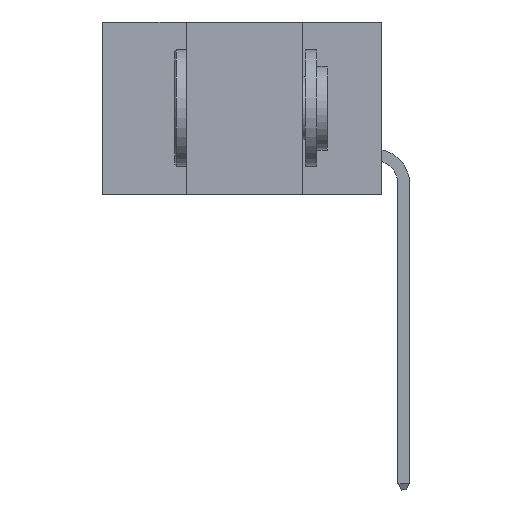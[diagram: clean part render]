
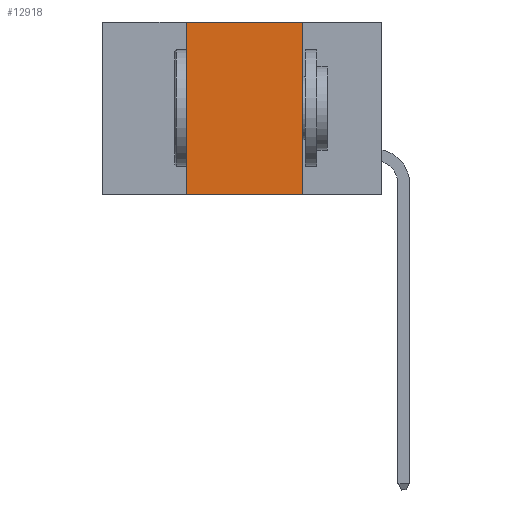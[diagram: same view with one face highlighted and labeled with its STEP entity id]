
A CAD part, left-side view. The second image highlights one B-rep face of the part: STEP entity #12918.
In plain terms, the highlighted planar face has unit normal (-1, 0, 0).
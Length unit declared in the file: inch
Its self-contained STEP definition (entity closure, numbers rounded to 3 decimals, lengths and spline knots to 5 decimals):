
#591 = DIRECTION ( 'NONE',  ( 0., -1., 0. ) ) ;
#1838 = EDGE_CURVE ( 'NONE', #25662, #21724, #28314, .T. ) ;
#2893 = VECTOR ( 'NONE', #22618, 39.37008 ) ;
#3326 = AXIS2_PLACEMENT_3D ( 'NONE', #33441, #36071, #27546 ) ;
#3823 = LINE ( 'NONE', #4662, #2893 ) ;
#4513 = ORIENTED_EDGE ( 'NONE', *, *, #1838, .F. ) ;
#4608 = CARTESIAN_POINT ( 'NONE',  ( 0., 0.6, -0.37 ) ) ;
#4662 = CARTESIAN_POINT ( 'NONE',  ( 0., 0.17, 0. ) ) ;
#4943 = ORIENTED_EDGE ( 'NONE', *, *, #9957, .F. ) ;
#5256 = EDGE_CURVE ( 'NONE', #9121, #16244, #3823, .T. ) ;
#6259 = DIRECTION ( 'NONE',  ( 0., 0., 1. ) ) ;
#9121 = VERTEX_POINT ( 'NONE', #31391 ) ;
#9957 = EDGE_CURVE ( 'NONE', #21724, #9121, #28969, .T. ) ;
#10278 = EDGE_CURVE ( 'NONE', #25662, #16244, #22866, .T. ) ;
#12918 = ADVANCED_FACE ( 'NONE', ( #18488 ), #15177, .F. ) ;
#12980 = CARTESIAN_POINT ( 'NONE',  ( 0., 0.6, 0. ) ) ;
#14425 = EDGE_LOOP ( 'NONE', ( #18119, #4943, #4513, #32311 ) ) ;
#14942 = VECTOR ( 'NONE', #16607, 39.37008 ) ;
#15177 = PLANE ( 'NONE',  #3326 ) ;
#16244 = VERTEX_POINT ( 'NONE', #32021 ) ;
#16607 = DIRECTION ( 'NONE',  ( 0., -1., 0. ) ) ;
#17312 = VECTOR ( 'NONE', #591, 39.37008 ) ;
#18119 = ORIENTED_EDGE ( 'NONE', *, *, #5256, .F. ) ;
#18488 = FACE_OUTER_BOUND ( 'NONE', #14425, .T. ) ;
#21724 = VERTEX_POINT ( 'NONE', #28855 ) ;
#22618 = DIRECTION ( 'NONE',  ( 0., 0., -1. ) ) ;
#22866 = LINE ( 'NONE', #4608, #14942 ) ;
#25662 = VERTEX_POINT ( 'NONE', #32627 ) ;
#27546 = DIRECTION ( 'NONE',  ( 0., 0., -1. ) ) ;
#28314 = LINE ( 'NONE', #32479, #38151 ) ;
#28855 = CARTESIAN_POINT ( 'NONE',  ( 0., 0.42, 0. ) ) ;
#28969 = LINE ( 'NONE', #12980, #17312 ) ;
#31391 = CARTESIAN_POINT ( 'NONE',  ( 0., 0.17, 0. ) ) ;
#32021 = CARTESIAN_POINT ( 'NONE',  ( 0., 0.17, -0.37 ) ) ;
#32311 = ORIENTED_EDGE ( 'NONE', *, *, #10278, .T. ) ;
#32479 = CARTESIAN_POINT ( 'NONE',  ( 0., 0.42, 0. ) ) ;
#32627 = CARTESIAN_POINT ( 'NONE',  ( 0., 0.42, -0.37 ) ) ;
#33441 = CARTESIAN_POINT ( 'NONE',  ( 0., 0.6, 0. ) ) ;
#36071 = DIRECTION ( 'NONE',  ( 1., 0., 0. ) ) ;
#38151 = VECTOR ( 'NONE', #6259, 39.37008 ) ;
